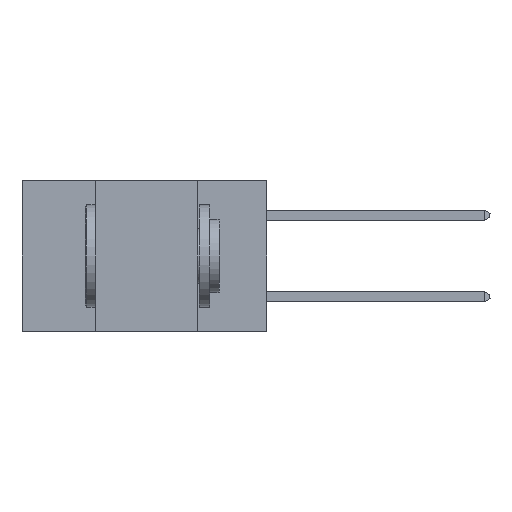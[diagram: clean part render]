
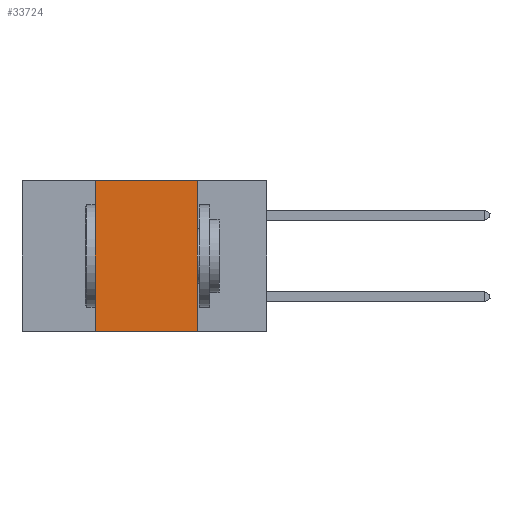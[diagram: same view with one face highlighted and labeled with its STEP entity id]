
A CAD part, left-side view. The second image highlights one B-rep face of the part: STEP entity #33724.
In plain terms, the highlighted planar face has unit normal (-1, 0, 0).
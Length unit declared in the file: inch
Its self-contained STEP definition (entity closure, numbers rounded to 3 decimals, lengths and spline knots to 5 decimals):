
#1095 = DIRECTION ( 'NONE',  ( 0., 0., -1. ) ) ;
#3199 = EDGE_LOOP ( 'NONE', ( #47750, #29307, #41496, #5467 ) ) ;
#3326 = CARTESIAN_POINT ( 'NONE',  ( 0., 0.42, 0. ) ) ;
#5467 = ORIENTED_EDGE ( 'NONE', *, *, #10376, .T. ) ;
#9560 = CARTESIAN_POINT ( 'NONE',  ( 0., 0.17, 0. ) ) ;
#10376 = EDGE_CURVE ( 'NONE', #34847, #21604, #47773, .T. ) ;
#10400 = CARTESIAN_POINT ( 'NONE',  ( 0., 0.6, -0.37 ) ) ;
#13355 = PLANE ( 'NONE',  #16742 ) ;
#13700 = FACE_OUTER_BOUND ( 'NONE', #3199, .T. ) ;
#14200 = DIRECTION ( 'NONE',  ( 0., -1., 0. ) ) ;
#14295 = CARTESIAN_POINT ( 'NONE',  ( 0., 0.42, 0. ) ) ;
#16742 = AXIS2_PLACEMENT_3D ( 'NONE', #46473, #39267, #17077 ) ;
#17077 = DIRECTION ( 'NONE',  ( 0., 0., -1. ) ) ;
#18015 = DIRECTION ( 'NONE',  ( 0., 0., 1. ) ) ;
#18331 = VECTOR ( 'NONE', #14200, 39.37008 ) ;
#19475 = DIRECTION ( 'NONE',  ( 0., -1., 0. ) ) ;
#21604 = VERTEX_POINT ( 'NONE', #45518 ) ;
#23064 = VECTOR ( 'NONE', #18015, 39.37008 ) ;
#25392 = LINE ( 'NONE', #14295, #23064 ) ;
#29307 = ORIENTED_EDGE ( 'NONE', *, *, #44201, .F. ) ;
#29354 = EDGE_CURVE ( 'NONE', #32158, #21604, #32288, .T. ) ;
#30384 = CARTESIAN_POINT ( 'NONE',  ( 0., 0.42, -0.37 ) ) ;
#31108 = VECTOR ( 'NONE', #1095, 39.37008 ) ;
#32158 = VERTEX_POINT ( 'NONE', #9560 ) ;
#32288 = LINE ( 'NONE', #45584, #31108 ) ;
#33724 = ADVANCED_FACE ( 'NONE', ( #13700 ), #13355, .F. ) ;
#34847 = VERTEX_POINT ( 'NONE', #30384 ) ;
#36656 = VERTEX_POINT ( 'NONE', #3326 ) ;
#39267 = DIRECTION ( 'NONE',  ( 1., 0., 0. ) ) ;
#41496 = ORIENTED_EDGE ( 'NONE', *, *, #42680, .F. ) ;
#41686 = CARTESIAN_POINT ( 'NONE',  ( 0., 0.6, 0. ) ) ;
#42680 = EDGE_CURVE ( 'NONE', #34847, #36656, #25392, .T. ) ;
#44201 = EDGE_CURVE ( 'NONE', #36656, #32158, #44983, .T. ) ;
#44983 = LINE ( 'NONE', #41686, #47270 ) ;
#45518 = CARTESIAN_POINT ( 'NONE',  ( 0., 0.17, -0.37 ) ) ;
#45584 = CARTESIAN_POINT ( 'NONE',  ( 0., 0.17, 0. ) ) ;
#46473 = CARTESIAN_POINT ( 'NONE',  ( 0., 0.6, 0. ) ) ;
#47270 = VECTOR ( 'NONE', #19475, 39.37008 ) ;
#47750 = ORIENTED_EDGE ( 'NONE', *, *, #29354, .F. ) ;
#47773 = LINE ( 'NONE', #10400, #18331 ) ;
